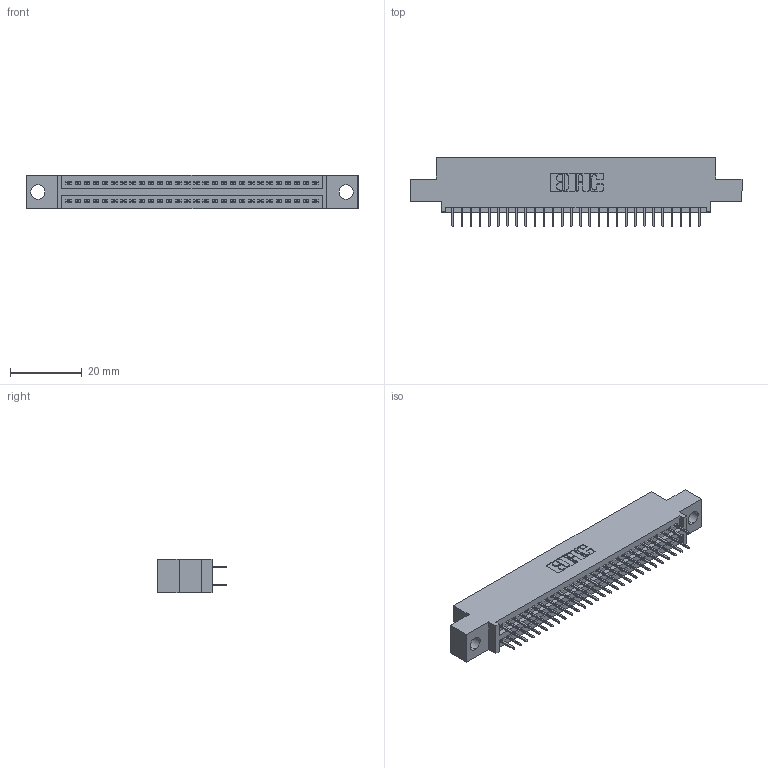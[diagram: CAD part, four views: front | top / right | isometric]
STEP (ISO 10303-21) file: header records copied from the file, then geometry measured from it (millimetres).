
FILE_DESCRIPTION (( 'STEP AP203' ), '1' );
FILE_NAME ('395-056-524-504.STEP', '2021-06-17T01:06:38', ( '' ), ( '' ), 'SwSTEP 2.0', 'SolidWorks 2020', '' );
FILE_SCHEMA (( 'CONFIG_CONTROL_DESIGN' ));
Length unit declared in the file: inch
Products named in the file (3): 395-056-524-504; 345-292-001_345-293-124; 345 Part_0.110 Offset - 0.156 Dia-TI
Assembly tree (57 placements, depth 2):
  395-056-524-504
    345 Part_0.110 Offset - 0.156 Dia-TI
    345-292-001_345-293-124  x56
Bounding box: 92.33 x 19.35 x 9.4 mm (x, y, z)
Volume: 8574.9 mm3; surface area: 12124.7 mm2
Topology: 57 solids, 57 shells, 3168 faces, 8957 edges, 5746 vertices
Faces by surface type: plane 2282, cylinder 886
Entity records: 24479 total; most frequent: CARTESIAN_POINT 4122, ORIENTED_EDGE 4054, DIRECTION 3651, EDGE_CURVE 2027, VECTOR 1787, LINE 1787, VERTEX_POINT 1346, AXIS2_PLACEMENT_3D 932
